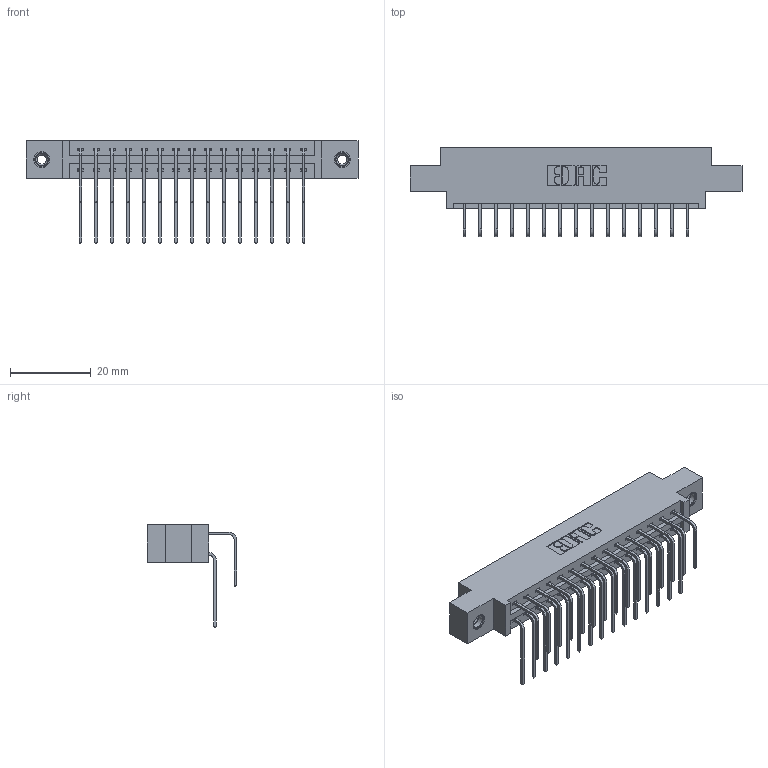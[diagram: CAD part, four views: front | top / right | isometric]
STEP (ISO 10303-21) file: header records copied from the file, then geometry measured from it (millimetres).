
FILE_DESCRIPTION (( 'STEP AP203' ), '1' );
FILE_NAME ('387-030-558-808.STEP', '2018-09-18T03:29:10', ( '' ), ( '' ), 'SwSTEP 2.0', 'SolidWorks 2016', '' );
FILE_SCHEMA (( 'CONFIG_CONTROL_DESIGN' ));
Length unit declared in the file: inch
Products named in the file (5): 337 Part_0.170 Offset - 0.156 Dia-TI; 345-292-001_558 559 Tail - 1; 345-292-001_558 Tail - 2; 345-250-001_345-250-003-102; 387-030-558-808
Assembly tree (33 placements, depth 2):
  387-030-558-808
    337 Part_0.170 Offset - 0.156 Dia-TI
    345-292-001_558 559 Tail - 1  x15
    345-292-001_558 Tail - 2  x15
    345-250-001_345-250-003-102  x2
Bounding box: 82.45 x 22.17 x 25.53 mm (x, y, z)
Volume: 8378.7 mm3; surface area: 10210.6 mm2
Topology: 33 solids, 33 shells, 1858 faces, 5469 edges, 3598 vertices
Faces by surface type: plane 1306, cylinder 536, cone 12, torus 4
Entity records: 18224 total; most frequent: CARTESIAN_POINT 3120, ORIENTED_EDGE 2998, DIRECTION 2717, EDGE_CURVE 1499, VECTOR 1311, LINE 1311, VERTEX_POINT 992, AXIS2_PLACEMENT_3D 703
